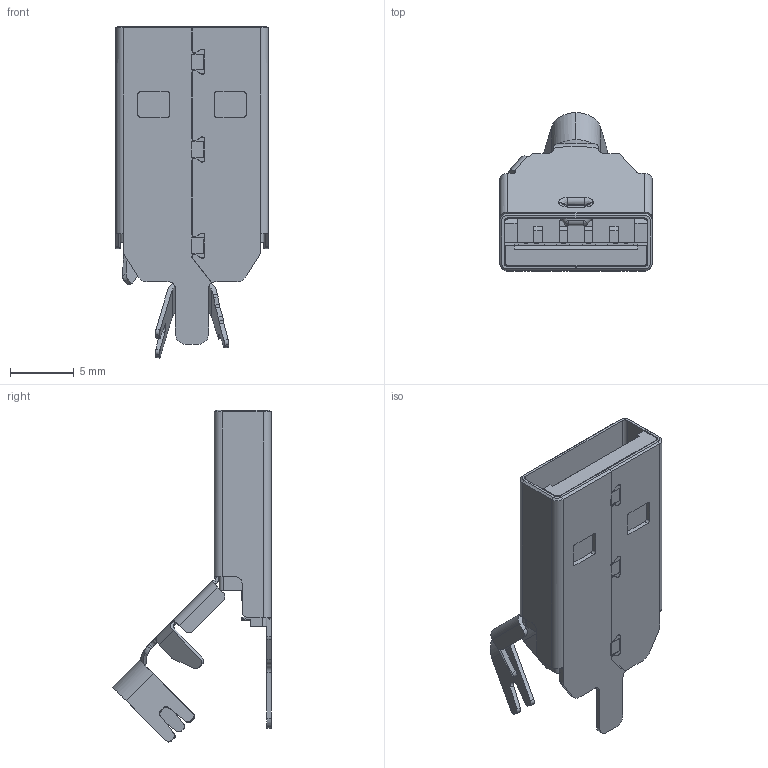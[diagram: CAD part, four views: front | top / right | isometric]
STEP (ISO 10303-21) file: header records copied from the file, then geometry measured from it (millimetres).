
FILE_DESCRIPTION (( 'STEP AP214' ), '1' );
FILE_NAME ('691E104P5A0-268.STEP', '2021-01-19T14:37:50', ( '' ), ( '' ), 'SwSTEP 2.0', 'SolidWorks 2020', '' );
FILE_SCHEMA (( 'AUTOMOTIVE_DESIGN' ));
Length unit declared in the file: millimetre
Products named in the file (7): PIN4 691E104P5A0-26X; PIN3 691E104P5A0-26X; 691E104P5A0-268; PIN2 691E104P5A0-26X; SHELL 691E104P5A0-26X_Open; PIN1 691E104P5A0-26X; HOUSING 691E104P5A0-26X_Grey
Assembly tree (6 placements, depth 2):
  691E104P5A0-268
    HOUSING 691E104P5A0-26X_Grey
    PIN1 691E104P5A0-26X
    PIN2 691E104P5A0-26X
    PIN3 691E104P5A0-26X
    PIN4 691E104P5A0-26X
    SHELL 691E104P5A0-26X_Open
Bounding box: 12 x 12.46 x 26.08 mm (x, y, z)
Volume: 568 mm3; surface area: 2323.6 mm2
Topology: 6 solids, 6 shells, 1302 faces, 3359 edges, 2162 vertices
Faces by surface type: plane 991, cylinder 237, bspline 62, cone 12
Entity records: 42648 total; most frequent: CARTESIAN_POINT 10937, ORIENTED_EDGE 6646, DIRECTION 6120, EDGE_CURVE 3323, LINE 2722, VECTOR 2722, VERTEX_POINT 2162, AXIS2_PLACEMENT_3D 1699
